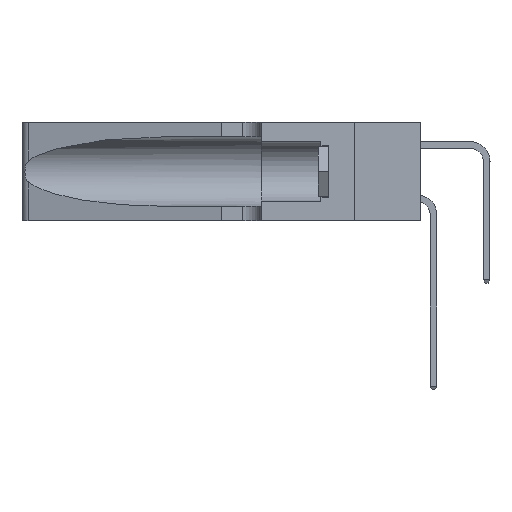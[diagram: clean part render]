
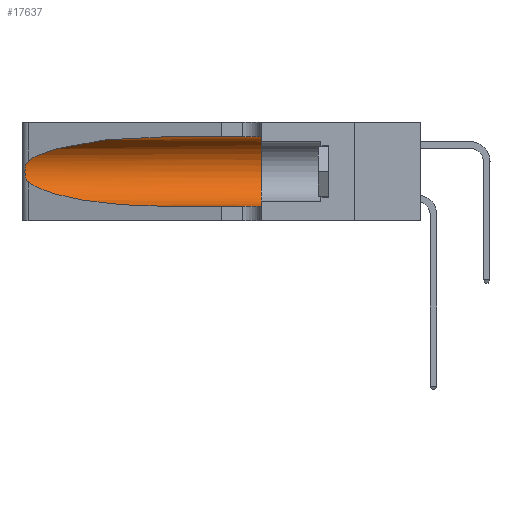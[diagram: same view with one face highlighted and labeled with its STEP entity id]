
A CAD part, left-side view. The second image highlights one B-rep face of the part: STEP entity #17637.
In plain terms, the highlighted cylindrical face has radius 3.308 mm (diameter 6.617 mm), a partial arc.
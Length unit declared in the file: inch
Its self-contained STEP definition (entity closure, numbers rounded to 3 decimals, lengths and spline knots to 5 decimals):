
#763 = ORIENTED_EDGE ( 'NONE', *, *, #36972, .T. ) ;
#1202 = VERTEX_POINT ( 'NONE', #13704 ) ;
#1732 = CARTESIAN_POINT ( 'NONE',  ( 0.1305, 0.72297, 0.05475 ) ) ;
#2812 = DIRECTION ( 'NONE',  ( 0., 0., 1. ) ) ;
#2838 = CARTESIAN_POINT ( 'NONE',  ( 0.25639, 1.23184, 0.21858 ) ) ;
#4126 = CARTESIAN_POINT ( 'NONE',  ( 0.1305, 0.35, 0.05475 ) ) ;
#5337 = CARTESIAN_POINT ( 'NONE',  ( 0.25487, 1.22718, 0.22369 ) ) ;
#5922 = CARTESIAN_POINT ( 'NONE',  ( 0.25854, 1.2359, 0.20912 ) ) ;
#7418 = EDGE_CURVE ( 'NONE', #26989, #7721, #32544, .T. ) ;
#7721 = VERTEX_POINT ( 'NONE', #4126 ) ;
#8364 = CARTESIAN_POINT ( 'NONE',  ( 0.25487, 1.22718, 0.14631 ) ) ;
#8943 = CARTESIAN_POINT ( 'NONE',  ( 0.26075, 1.23896, 0.19203 ) ) ;
#9823 = VERTEX_POINT ( 'NONE', #36102 ) ;
#10093 = ORIENTED_EDGE ( 'NONE', *, *, #35956, .T. ) ;
#10323 = VECTOR ( 'NONE', #35806, 39.37008 ) ;
#10504 = CARTESIAN_POINT ( 'NONE',  ( 0.1305, 0.35, 0.31525 ) ) ;
#10819 = DIRECTION ( 'NONE',  ( 0., 0., -1. ) ) ;
#11931 = CARTESIAN_POINT ( 'NONE',  ( 0.26017, 1.23833, 0.17102 ) ) ;
#13704 = CARTESIAN_POINT ( 'NONE',  ( 0.25487, 1.22718, 0.22369 ) ) ;
#14034 = ORIENTED_EDGE ( 'NONE', *, *, #7418, .F. ) ;
#14990 = CARTESIAN_POINT ( 'NONE',  ( 0.25789, 1.23486, 0.15765 ) ) ;
#15586 = CARTESIAN_POINT ( 'NONE',  ( 0.1305, 1.61858, 0.31525 ) ) ;
#17637 = ADVANCED_FACE ( 'NONE', ( #32632 ), #31707, .F. ) ;
#17772 = VECTOR ( 'NONE', #18552, 39.37008 ) ;
#17789 =( BOUNDED_CURVE ( )  B_SPLINE_CURVE ( 3, ( #38022, #20262, #23259, #5337 ),
 .UNSPECIFIED., .F., .F. ) 
 B_SPLINE_CURVE_WITH_KNOTS ( ( 4, 4 ),
 ( 1.5708, 2.84003 ),
 .UNSPECIFIED. ) 
 CURVE ( )  GEOMETRIC_REPRESENTATION_ITEM ( )  RATIONAL_B_SPLINE_CURVE ( ( 1., 0.87, 0.87, 1. ) ) 
 REPRESENTATION_ITEM ( '' )  );
#17845 = CARTESIAN_POINT ( 'NONE',  ( 0.25487, 1.22718, 0.22369 ) ) ;
#17968 = CARTESIAN_POINT ( 'NONE',  ( 0.25555, 1.22993, 0.14849 ) ) ;
#18552 = DIRECTION ( 'NONE',  ( 0., -1., 0. ) ) ;
#18969 = VERTEX_POINT ( 'NONE', #8364 ) ;
#19742 = EDGE_LOOP ( 'NONE', ( #25226, #28988, #763, #10093, #14034, #20178 ) ) ;
#19759 = CARTESIAN_POINT ( 'NONE',  ( 0.18966, 0.96281, 0.05475 ) ) ;
#20178 = ORIENTED_EDGE ( 'NONE', *, *, #37369, .F. ) ;
#20262 = CARTESIAN_POINT ( 'NONE',  ( 0.18966, 0.96281, 0.31525 ) ) ;
#20811 = DIRECTION ( 'NONE',  ( 0., 1., 0. ) ) ;
#20843 = CARTESIAN_POINT ( 'NONE',  ( 0.25555, 1.22994, 0.2215 ) ) ;
#21843 =( BOUNDED_CURVE ( )  B_SPLINE_CURVE ( 3, ( #28603, #25606, #19759, #1732 ),
 .UNSPECIFIED., .F., .F. ) 
 B_SPLINE_CURVE_WITH_KNOTS ( ( 4, 4 ),
 ( 3.44316, 4.71239 ),
 .UNSPECIFIED. ) 
 CURVE ( )  GEOMETRIC_REPRESENTATION_ITEM ( )  RATIONAL_B_SPLINE_CURVE ( ( 1., 0.87, 0.87, 1. ) ) 
 REPRESENTATION_ITEM ( '' )  );
#23259 = CARTESIAN_POINT ( 'NONE',  ( 0.2373, 1.15595, 0.28018 ) ) ;
#23838 = CARTESIAN_POINT ( 'NONE',  ( 0.25787, 1.23484, 0.2124 ) ) ;
#24719 = EDGE_CURVE ( 'NONE', #1202, #18969, #38481, .T. ) ;
#25226 = ORIENTED_EDGE ( 'NONE', *, *, #29669, .T. ) ;
#25606 = CARTESIAN_POINT ( 'NONE',  ( 0.2373, 1.15595, 0.08982 ) ) ;
#25805 = DIRECTION ( 'NONE',  ( 0., -1., 0. ) ) ;
#26616 = LINE ( 'NONE', #15586, #17772 ) ;
#26825 = CARTESIAN_POINT ( 'NONE',  ( 0.26018, 1.23835, 0.19895 ) ) ;
#26989 = VERTEX_POINT ( 'NONE', #10504 ) ;
#28603 = CARTESIAN_POINT ( 'NONE',  ( 0.25487, 1.22718, 0.14631 ) ) ;
#28747 = AXIS2_PLACEMENT_3D ( 'NONE', #38568, #20811, #2812 ) ;
#28988 = ORIENTED_EDGE ( 'NONE', *, *, #24719, .T. ) ;
#29669 = EDGE_CURVE ( 'NONE', #35341, #1202, #17789, .T. ) ;
#29817 = CARTESIAN_POINT ( 'NONE',  ( 0.26075, 1.23896, 0.178 ) ) ;
#30340 = AXIS2_PLACEMENT_3D ( 'NONE', #31684, #25805, #10819 ) ;
#31684 = CARTESIAN_POINT ( 'NONE',  ( 0.1305, 1.61858, 0.185 ) ) ;
#31707 = CYLINDRICAL_SURFACE ( 'NONE', #30340, 0.13025 ) ;
#32544 = CIRCLE ( 'NONE', #28747, 0.13025 ) ;
#32632 = FACE_OUTER_BOUND ( 'NONE', #19742, .T. ) ;
#32798 = CARTESIAN_POINT ( 'NONE',  ( 0.25856, 1.23593, 0.16098 ) ) ;
#32837 = CARTESIAN_POINT ( 'NONE',  ( 0.1305, 1.61858, 0.05475 ) ) ;
#33343 = CARTESIAN_POINT ( 'NONE',  ( 0.1305, 0.72297, 0.31525 ) ) ;
#34099 = LINE ( 'NONE', #32837, #10323 ) ;
#35341 = VERTEX_POINT ( 'NONE', #33343 ) ;
#35761 = CARTESIAN_POINT ( 'NONE',  ( 0.25639, 1.23186, 0.15144 ) ) ;
#35806 = DIRECTION ( 'NONE',  ( 0., -1., 0. ) ) ;
#35956 = EDGE_CURVE ( 'NONE', #9823, #7721, #34099, .T. ) ;
#36102 = CARTESIAN_POINT ( 'NONE',  ( 0.1305, 0.72297, 0.05475 ) ) ;
#36972 = EDGE_CURVE ( 'NONE', #18969, #9823, #21843, .T. ) ;
#37369 = EDGE_CURVE ( 'NONE', #35341, #26989, #26616, .T. ) ;
#38022 = CARTESIAN_POINT ( 'NONE',  ( 0.1305, 0.72297, 0.31525 ) ) ;
#38481 = B_SPLINE_CURVE_WITH_KNOTS ( 'NONE', 3,
 ( #17845, #20843, #2838, #23838, #5922, #26825, #8943, #29817, #11931, #32798, #14990, #35761, #17968, #38731 ),
 .UNSPECIFIED., .F., .F.,
 ( 4, 2, 2, 2, 2, 2, 4 ),
 ( 0., 0.00027, 0.00053, 0.00107, 0.0016, 0.00187, 0.00214 ),
 .UNSPECIFIED. ) ;
#38568 = CARTESIAN_POINT ( 'NONE',  ( 0.1305, 0.35, 0.185 ) ) ;
#38731 = CARTESIAN_POINT ( 'NONE',  ( 0.25487, 1.22718, 0.14631 ) ) ;
